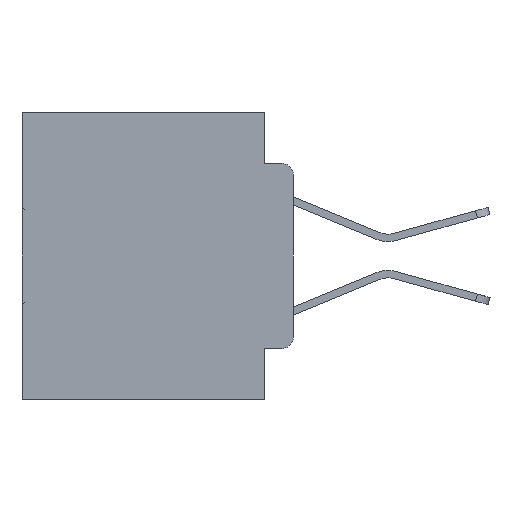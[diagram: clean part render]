
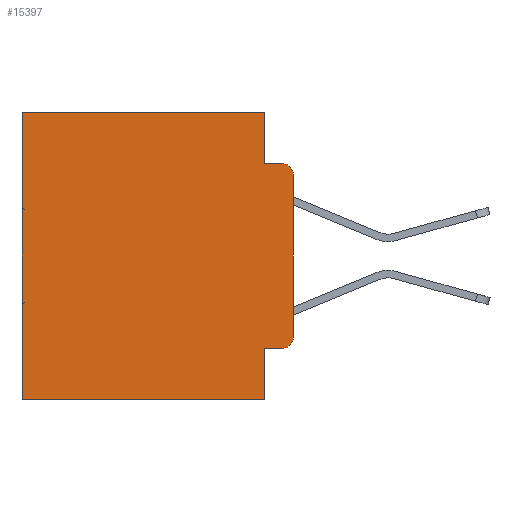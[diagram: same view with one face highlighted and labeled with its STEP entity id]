
A CAD part, left-side view. The second image highlights one B-rep face of the part: STEP entity #15397.
In plain terms, the highlighted planar face has unit normal (-1, 0, 0).
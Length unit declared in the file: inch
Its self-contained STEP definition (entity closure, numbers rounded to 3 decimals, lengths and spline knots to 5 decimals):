
#358 = CIRCLE ( 'NONE', #8407, 0.02 ) ;
#1517 = VECTOR ( 'NONE', #22571, 39.37008 ) ;
#1542 = ORIENTED_EDGE ( 'NONE', *, *, #31961, .T. ) ;
#2362 = CARTESIAN_POINT ( 'NONE',  ( 0.298, 0., -0.5 ) ) ;
#2371 = CARTESIAN_POINT ( 'NONE',  ( 0.298, 0.473, 0. ) ) ;
#2561 = VERTEX_POINT ( 'NONE', #8569 ) ;
#2918 = VECTOR ( 'NONE', #22639, 39.37008 ) ;
#3617 = ORIENTED_EDGE ( 'NONE', *, *, #29323, .T. ) ;
#3754 = CARTESIAN_POINT ( 'NONE',  ( 0.298, 0.051, 0. ) ) ;
#4764 = CARTESIAN_POINT ( 'NONE',  ( 0.298, 0., 0. ) ) ;
#4954 = FACE_OUTER_BOUND ( 'NONE', #19851, .T. ) ;
#5362 = VERTEX_POINT ( 'NONE', #13972 ) ;
#5579 = VERTEX_POINT ( 'NONE', #27249 ) ;
#5773 = CARTESIAN_POINT ( 'NONE',  ( 0.298, 0., -0.3915 ) ) ;
#5790 = DIRECTION ( 'NONE',  ( 0., 0., -1. ) ) ;
#6550 = ORIENTED_EDGE ( 'NONE', *, *, #12677, .F. ) ;
#7265 = VERTEX_POINT ( 'NONE', #30006 ) ;
#8167 = VERTEX_POINT ( 'NONE', #31020 ) ;
#8407 = AXIS2_PLACEMENT_3D ( 'NONE', #28231, #31187, #18660 ) ;
#8569 = CARTESIAN_POINT ( 'NONE',  ( 0.298, 0.02, -0.4115 ) ) ;
#9843 = VERTEX_POINT ( 'NONE', #11689 ) ;
#10308 = VERTEX_POINT ( 'NONE', #5773 ) ;
#10779 = CARTESIAN_POINT ( 'NONE',  ( 0.298, 0.02, -0.1085 ) ) ;
#10974 = VECTOR ( 'NONE', #27950, 39.37008 ) ;
#10999 = DIRECTION ( 'NONE',  ( 0., 0., -1. ) ) ;
#11689 = CARTESIAN_POINT ( 'NONE',  ( 0.298, 0.051, -0.5 ) ) ;
#11759 = LINE ( 'NONE', #4764, #1517 ) ;
#11786 = EDGE_CURVE ( 'NONE', #5362, #29166, #32167, .T. ) ;
#11957 = EDGE_CURVE ( 'NONE', #18730, #5579, #18445, .T. ) ;
#12677 = EDGE_CURVE ( 'NONE', #9843, #5579, #27879, .T. ) ;
#13221 = DIRECTION ( 'NONE',  ( 0., 0., -1. ) ) ;
#13566 = VECTOR ( 'NONE', #5790, 39.37008 ) ;
#13972 = CARTESIAN_POINT ( 'NONE',  ( 0.298, 0., -0.1085 ) ) ;
#14242 = VECTOR ( 'NONE', #25284, 39.37008 ) ;
#14303 = ORIENTED_EDGE ( 'NONE', *, *, #18011, .T. ) ;
#14546 = EDGE_CURVE ( 'NONE', #7265, #9843, #28113, .T. ) ;
#14868 = ORIENTED_EDGE ( 'NONE', *, *, #29191, .F. ) ;
#14920 = CARTESIAN_POINT ( 'NONE',  ( 0.298, 0.051, -0.0885 ) ) ;
#15397 = ADVANCED_FACE ( 'NONE', ( #4954 ), #25751, .F. ) ;
#15759 = VECTOR ( 'NONE', #30364, 39.37008 ) ;
#17673 = ORIENTED_EDGE ( 'NONE', *, *, #20692, .F. ) ;
#17715 = LINE ( 'NONE', #27761, #15759 ) ;
#18011 = EDGE_CURVE ( 'NONE', #2561, #10308, #358, .T. ) ;
#18445 = LINE ( 'NONE', #24082, #31029 ) ;
#18660 = DIRECTION ( 'NONE',  ( 0., 0., -1. ) ) ;
#18730 = VERTEX_POINT ( 'NONE', #2371 ) ;
#19851 = EDGE_LOOP ( 'NONE', ( #17673, #25483, #28621, #14868, #3617, #32533, #6550, #25655, #1542, #14303 ) ) ;
#20298 = AXIS2_PLACEMENT_3D ( 'NONE', #10779, #20668, #23436 ) ;
#20668 = DIRECTION ( 'NONE',  ( -1., 0., 0. ) ) ;
#20692 = EDGE_CURVE ( 'NONE', #5362, #10308, #11759, .T. ) ;
#22571 = DIRECTION ( 'NONE',  ( 0., 0., -1. ) ) ;
#22639 = DIRECTION ( 'NONE',  ( 0., -1., 0. ) ) ;
#22885 = VECTOR ( 'NONE', #10999, 39.37008 ) ;
#23436 = DIRECTION ( 'NONE',  ( 0., 0., -1. ) ) ;
#23484 = EDGE_CURVE ( 'NONE', #8167, #29166, #27719, .T. ) ;
#23551 = CARTESIAN_POINT ( 'NONE',  ( 0.298, 0.02, -0.0885 ) ) ;
#24082 = CARTESIAN_POINT ( 'NONE',  ( 0.298, 0.473, 0. ) ) ;
#24275 = CARTESIAN_POINT ( 'NONE',  ( 0.298, 0.051, 0. ) ) ;
#24601 = AXIS2_PLACEMENT_3D ( 'NONE', #30652, #28249, #13221 ) ;
#25284 = DIRECTION ( 'NONE',  ( 0., -1., 0. ) ) ;
#25483 = ORIENTED_EDGE ( 'NONE', *, *, #11786, .T. ) ;
#25655 = ORIENTED_EDGE ( 'NONE', *, *, #14546, .F. ) ;
#25751 = PLANE ( 'NONE',  #24601 ) ;
#26016 = CARTESIAN_POINT ( 'NONE',  ( 0.298, 0.051, 0. ) ) ;
#26408 = LINE ( 'NONE', #27377, #14242 ) ;
#26609 = DIRECTION ( 'NONE',  ( 0., 0., -1. ) ) ;
#27249 = CARTESIAN_POINT ( 'NONE',  ( 0.298, 0.473, -0.5 ) ) ;
#27377 = CARTESIAN_POINT ( 'NONE',  ( 0.298, 0.051, -0.4115 ) ) ;
#27719 = LINE ( 'NONE', #14920, #2918 ) ;
#27761 = CARTESIAN_POINT ( 'NONE',  ( 0.298, 0., 0. ) ) ;
#27879 = LINE ( 'NONE', #2362, #10974 ) ;
#27899 = VERTEX_POINT ( 'NONE', #24275 ) ;
#27950 = DIRECTION ( 'NONE',  ( 0., 1., 0. ) ) ;
#28113 = LINE ( 'NONE', #26016, #13566 ) ;
#28231 = CARTESIAN_POINT ( 'NONE',  ( 0.298, 0.02, -0.3915 ) ) ;
#28249 = DIRECTION ( 'NONE',  ( 1., 0., 0. ) ) ;
#28621 = ORIENTED_EDGE ( 'NONE', *, *, #23484, .F. ) ;
#29166 = VERTEX_POINT ( 'NONE', #23551 ) ;
#29191 = EDGE_CURVE ( 'NONE', #27899, #8167, #29550, .T. ) ;
#29323 = EDGE_CURVE ( 'NONE', #27899, #18730, #17715, .T. ) ;
#29550 = LINE ( 'NONE', #3754, #22885 ) ;
#30006 = CARTESIAN_POINT ( 'NONE',  ( 0.298, 0.051, -0.4115 ) ) ;
#30364 = DIRECTION ( 'NONE',  ( 0., 1., 0. ) ) ;
#30652 = CARTESIAN_POINT ( 'NONE',  ( 0.298, 0., 0. ) ) ;
#31020 = CARTESIAN_POINT ( 'NONE',  ( 0.298, 0.051, -0.0885 ) ) ;
#31029 = VECTOR ( 'NONE', #26609, 39.37008 ) ;
#31187 = DIRECTION ( 'NONE',  ( -1., 0., 0. ) ) ;
#31961 = EDGE_CURVE ( 'NONE', #7265, #2561, #26408, .T. ) ;
#32167 = CIRCLE ( 'NONE', #20298, 0.02 ) ;
#32533 = ORIENTED_EDGE ( 'NONE', *, *, #11957, .T. ) ;
